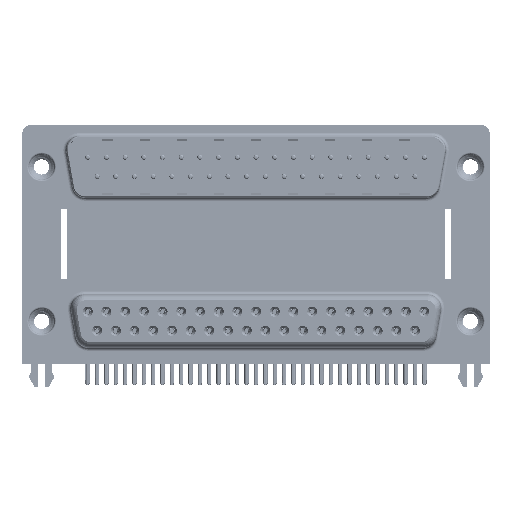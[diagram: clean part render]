
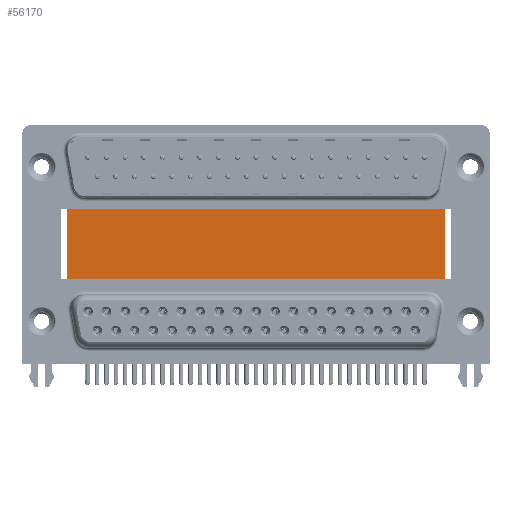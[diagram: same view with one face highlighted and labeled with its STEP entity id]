
A CAD part, top view. The second image highlights one B-rep face of the part: STEP entity #56170.
In plain terms, the highlighted planar face has unit normal (0, 0, 1).
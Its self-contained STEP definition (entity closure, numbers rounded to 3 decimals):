
#5311 = DIRECTION ( 'NONE',  ( 0., 0., -1. ) ) ;
#5900 = VECTOR ( 'NONE', #39332, 1000. ) ;
#7734 = EDGE_CURVE ( 'NONE', #53867, #61717, #10072, .T. ) ;
#8989 = DIRECTION ( 'NONE',  ( 1., 0., 0. ) ) ;
#9997 = CARTESIAN_POINT ( 'NONE',  ( 59.71, 16.585, -12. ) ) ;
#10072 = LINE ( 'NONE', #17093, #48663 ) ;
#10152 = CARTESIAN_POINT ( 'NONE',  ( 3.79, -3.735, -12. ) ) ;
#12451 = DIRECTION ( 'NONE',  ( 0., -1., 0. ) ) ;
#14441 = CARTESIAN_POINT ( 'NONE',  ( 59.71, -3.735, -12. ) ) ;
#15228 = ORIENTED_EDGE ( 'NONE', *, *, #42832, .F. ) ;
#17093 = CARTESIAN_POINT ( 'NONE',  ( 3.79, 16.585, -12. ) ) ;
#18223 = LINE ( 'NONE', #39680, #5900 ) ;
#18455 = VECTOR ( 'NONE', #8989, 1000. ) ;
#19990 = ORIENTED_EDGE ( 'NONE', *, *, #7734, .F. ) ;
#22064 = CARTESIAN_POINT ( 'NONE',  ( 3.79, 16.585, -12. ) ) ;
#23538 = ORIENTED_EDGE ( 'NONE', *, *, #30370, .T. ) ;
#27265 = DIRECTION ( 'NONE',  ( 1., 0., 0. ) ) ;
#28425 = VERTEX_POINT ( 'NONE', #14441 ) ;
#28738 = EDGE_CURVE ( 'NONE', #53867, #61354, #18223, .T. ) ;
#30370 = EDGE_CURVE ( 'NONE', #61354, #28425, #50874, .T. ) ;
#32426 = EDGE_LOOP ( 'NONE', ( #23538, #15228, #19990, #34061 ) ) ;
#33532 = CARTESIAN_POINT ( 'NONE',  ( 59.71, 16.585, -12. ) ) ;
#34061 = ORIENTED_EDGE ( 'NONE', *, *, #28738, .T. ) ;
#34660 = CARTESIAN_POINT ( 'NONE',  ( 3.79, -3.735, -12. ) ) ;
#37044 = AXIS2_PLACEMENT_3D ( 'NONE', #65805, #5311, #53543 ) ;
#37681 = FACE_OUTER_BOUND ( 'NONE', #32426, .T. ) ;
#38218 = LINE ( 'NONE', #33532, #46583 ) ;
#39332 = DIRECTION ( 'NONE',  ( 0., -1., 0. ) ) ;
#39680 = CARTESIAN_POINT ( 'NONE',  ( 3.79, 16.585, -12. ) ) ;
#42832 = EDGE_CURVE ( 'NONE', #61717, #28425, #38218, .T. ) ;
#43651 = PLANE ( 'NONE',  #37044 ) ;
#46583 = VECTOR ( 'NONE', #12451, 1000. ) ;
#48663 = VECTOR ( 'NONE', #27265, 1000. ) ;
#50874 = LINE ( 'NONE', #34660, #18455 ) ;
#53543 = DIRECTION ( 'NONE',  ( -1., 0., 0. ) ) ;
#53867 = VERTEX_POINT ( 'NONE', #22064 ) ;
#56170 = ADVANCED_FACE ( 'NONE', ( #37681 ), #43651, .F. ) ;
#61354 = VERTEX_POINT ( 'NONE', #10152 ) ;
#61717 = VERTEX_POINT ( 'NONE', #9997 ) ;
#65805 = CARTESIAN_POINT ( 'NONE',  ( 3.79, 16.585, -12. ) ) ;
